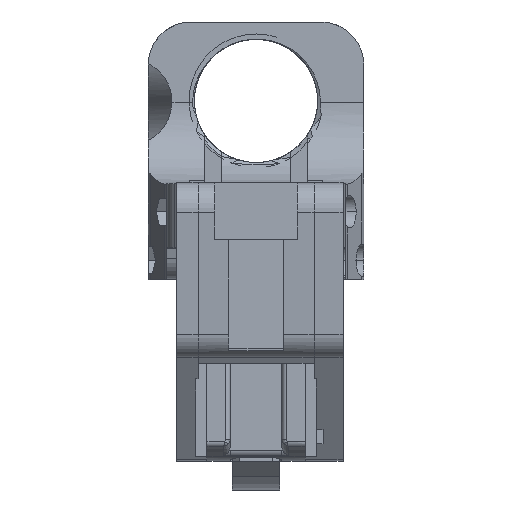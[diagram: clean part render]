
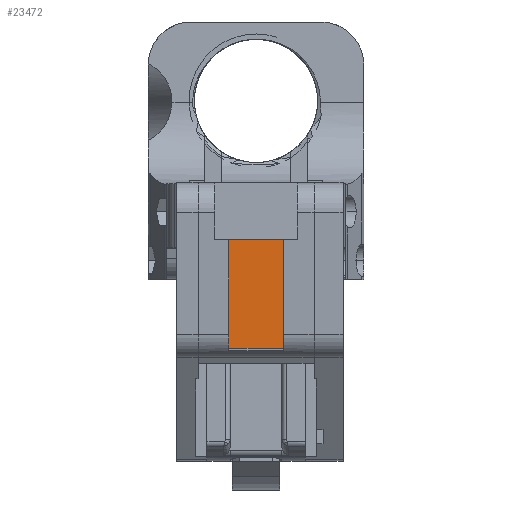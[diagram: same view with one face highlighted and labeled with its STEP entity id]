
A CAD part, top view. The second image highlights one B-rep face of the part: STEP entity #23472.
In plain terms, the highlighted face is planar.
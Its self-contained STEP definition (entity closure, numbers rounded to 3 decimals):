
#160 = VECTOR ( 'NONE', #3208, 1000. ) ;
#837 = CARTESIAN_POINT ( 'NONE',  ( -33.027, -38.329, 2.5 ) ) ;
#1864 = DIRECTION ( 'NONE',  ( 1., 0., 0. ) ) ;
#1977 = CARTESIAN_POINT ( 'NONE',  ( -6.35, -13.192, 2.5 ) ) ;
#3208 = DIRECTION ( 'NONE',  ( -1., 0., 0. ) ) ;
#4960 = VERTEX_POINT ( 'NONE', #1977 ) ;
#9460 = CARTESIAN_POINT ( 'NONE',  ( 6.35, -13.192, 2.5 ) ) ;
#12660 = DIRECTION ( 'NONE',  ( 1., 0., 0. ) ) ;
#13458 = DIRECTION ( 'NONE',  ( 0., -1., 0. ) ) ;
#13878 = AXIS2_PLACEMENT_3D ( 'NONE', #52130, #68044, #1864 ) ;
#17169 = ORIENTED_EDGE ( 'NONE', *, *, #65730, .F. ) ;
#17186 = EDGE_CURVE ( 'NONE', #50758, #48296, #46280, .T. ) ;
#23472 = ADVANCED_FACE ( 'NONE', ( #45466 ), #28511, .F. ) ;
#25076 = CARTESIAN_POINT ( 'NONE',  ( -6.35, -38.329, 2.5 ) ) ;
#28511 = PLANE ( 'NONE',  #13878 ) ;
#32391 = LINE ( 'NONE', #9460, #160 ) ;
#32464 = DIRECTION ( 'NONE',  ( 0., 1., 0. ) ) ;
#33456 = VECTOR ( 'NONE', #32464, 1000. ) ;
#36170 = EDGE_LOOP ( 'NONE', ( #65224, #65431, #17169, #42186 ) ) ;
#37994 = CARTESIAN_POINT ( 'NONE',  ( 6.35, -38.329, 2.5 ) ) ;
#39055 = CARTESIAN_POINT ( 'NONE',  ( 6.35, -38.329, 2.5 ) ) ;
#39722 = EDGE_CURVE ( 'NONE', #4960, #50758, #41538, .T. ) ;
#41538 = LINE ( 'NONE', #58193, #61173 ) ;
#41639 = VECTOR ( 'NONE', #12660, 1000. ) ;
#42186 = ORIENTED_EDGE ( 'NONE', *, *, #17186, .F. ) ;
#43875 = LINE ( 'NONE', #37994, #33456 ) ;
#45466 = FACE_OUTER_BOUND ( 'NONE', #36170, .T. ) ;
#46280 = LINE ( 'NONE', #837, #41639 ) ;
#48296 = VERTEX_POINT ( 'NONE', #39055 ) ;
#50084 = CARTESIAN_POINT ( 'NONE',  ( 6.35, -13.192, 2.5 ) ) ;
#50758 = VERTEX_POINT ( 'NONE', #25076 ) ;
#52130 = CARTESIAN_POINT ( 'NONE',  ( -33.027, -38.329, 2.5 ) ) ;
#55994 = EDGE_CURVE ( 'NONE', #57645, #4960, #32391, .T. ) ;
#57645 = VERTEX_POINT ( 'NONE', #50084 ) ;
#58193 = CARTESIAN_POINT ( 'NONE',  ( -6.35, -38.329, 2.5 ) ) ;
#61173 = VECTOR ( 'NONE', #13458, 1000. ) ;
#65224 = ORIENTED_EDGE ( 'NONE', *, *, #39722, .F. ) ;
#65431 = ORIENTED_EDGE ( 'NONE', *, *, #55994, .F. ) ;
#65730 = EDGE_CURVE ( 'NONE', #48296, #57645, #43875, .T. ) ;
#68044 = DIRECTION ( 'NONE',  ( 0., 0., 1. ) ) ;
